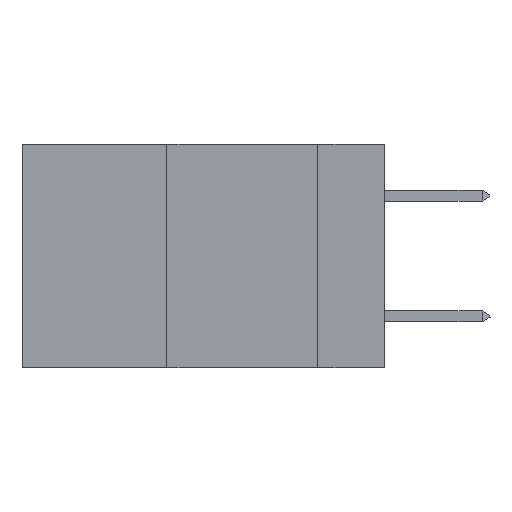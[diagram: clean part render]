
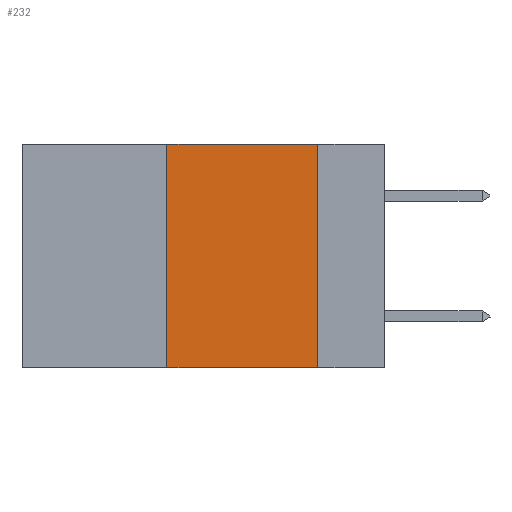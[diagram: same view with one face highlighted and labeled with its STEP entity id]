
A CAD part, left-side view. The second image highlights one B-rep face of the part: STEP entity #232.
In plain terms, the highlighted planar face has unit normal (-1, 0, 0).
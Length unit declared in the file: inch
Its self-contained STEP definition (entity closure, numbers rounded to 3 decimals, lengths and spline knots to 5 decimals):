
#204 = DIRECTION ( 'NONE',  ( 0., -1., 0. ) ) ;
#232 = ADVANCED_FACE ( 'NONE', ( #17005 ), #19747, .F. ) ;
#1479 = EDGE_CURVE ( 'NONE', #14292, #8578, #13790, .T. ) ;
#1587 = VECTOR ( 'NONE', #204, 39.37008 ) ;
#2041 = VECTOR ( 'NONE', #7568, 39.37008 ) ;
#3576 = ORIENTED_EDGE ( 'NONE', *, *, #25111, .F. ) ;
#5404 = CARTESIAN_POINT ( 'NONE',  ( 0., 0.11, 0. ) ) ;
#6473 = CARTESIAN_POINT ( 'NONE',  ( 0., 0.36, 0. ) ) ;
#7003 = CARTESIAN_POINT ( 'NONE',  ( 0., 0.11, -0.37 ) ) ;
#7097 = VECTOR ( 'NONE', #11658, 39.37008 ) ;
#7568 = DIRECTION ( 'NONE',  ( 0., -1., 0. ) ) ;
#7674 = LINE ( 'NONE', #6473, #23556 ) ;
#8578 = VERTEX_POINT ( 'NONE', #7003 ) ;
#8771 = EDGE_CURVE ( 'NONE', #14080, #8578, #15144, .T. ) ;
#9108 = DIRECTION ( 'NONE',  ( 1., 0., 0. ) ) ;
#9394 = ORIENTED_EDGE ( 'NONE', *, *, #1479, .T. ) ;
#11658 = DIRECTION ( 'NONE',  ( 0., 0., -1. ) ) ;
#12815 = CARTESIAN_POINT ( 'NONE',  ( 0., 0.11, 0. ) ) ;
#13790 = LINE ( 'NONE', #14207, #2041 ) ;
#14080 = VERTEX_POINT ( 'NONE', #12815 ) ;
#14207 = CARTESIAN_POINT ( 'NONE',  ( 0., 0.6, -0.37 ) ) ;
#14292 = VERTEX_POINT ( 'NONE', #19708 ) ;
#14527 = VERTEX_POINT ( 'NONE', #16484 ) ;
#14995 = DIRECTION ( 'NONE',  ( 0., 0., 1. ) ) ;
#15144 = LINE ( 'NONE', #5404, #7097 ) ;
#15235 = CARTESIAN_POINT ( 'NONE',  ( 0., 0.6, 0. ) ) ;
#16484 = CARTESIAN_POINT ( 'NONE',  ( 0., 0.36, 0. ) ) ;
#17005 = FACE_OUTER_BOUND ( 'NONE', #24869, .T. ) ;
#18400 = ORIENTED_EDGE ( 'NONE', *, *, #8771, .F. ) ;
#18758 = LINE ( 'NONE', #15235, #1587 ) ;
#19708 = CARTESIAN_POINT ( 'NONE',  ( 0., 0.36, -0.37 ) ) ;
#19747 = PLANE ( 'NONE',  #24915 ) ;
#19934 = DIRECTION ( 'NONE',  ( 0., 0., -1. ) ) ;
#22193 = CARTESIAN_POINT ( 'NONE',  ( 0., 0.6, 0. ) ) ;
#23556 = VECTOR ( 'NONE', #14995, 39.37008 ) ;
#24869 = EDGE_LOOP ( 'NONE', ( #18400, #25686, #3576, #9394 ) ) ;
#24915 = AXIS2_PLACEMENT_3D ( 'NONE', #22193, #9108, #19934 ) ;
#25111 = EDGE_CURVE ( 'NONE', #14292, #14527, #7674, .T. ) ;
#25686 = ORIENTED_EDGE ( 'NONE', *, *, #27466, .F. ) ;
#27466 = EDGE_CURVE ( 'NONE', #14527, #14080, #18758, .T. ) ;
